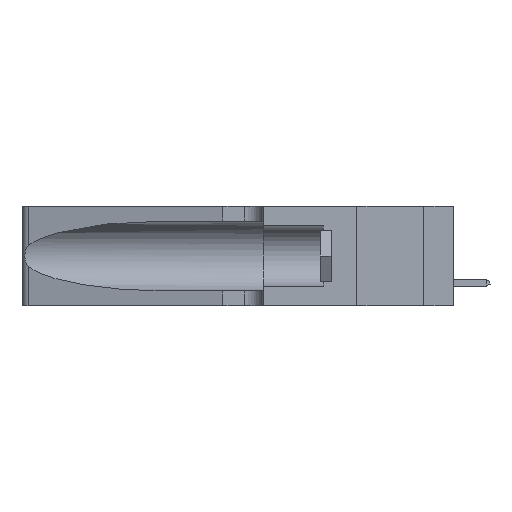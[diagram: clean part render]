
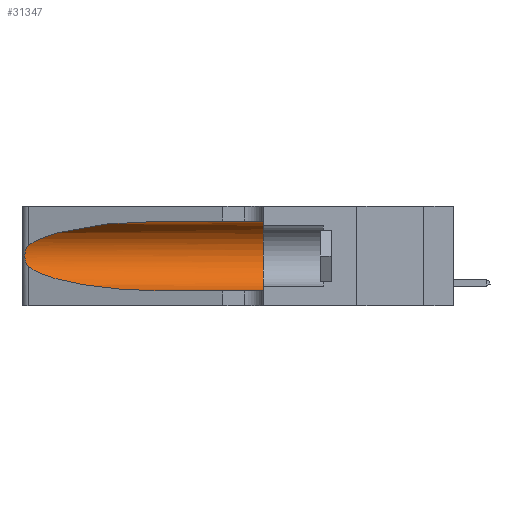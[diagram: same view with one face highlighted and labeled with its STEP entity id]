
A CAD part, left-side view. The second image highlights one B-rep face of the part: STEP entity #31347.
In plain terms, the highlighted cylindrical face has radius 3.308 mm (diameter 6.617 mm), a partial arc.
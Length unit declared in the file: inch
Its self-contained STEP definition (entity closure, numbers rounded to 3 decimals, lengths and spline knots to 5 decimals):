
#149 = CARTESIAN_POINT ( 'NONE',  ( 0.18966, 0.96281, 0.05475 ) ) ;
#315 = ORIENTED_EDGE ( 'NONE', *, *, #3881, .T. ) ;
#661 = CARTESIAN_POINT ( 'NONE',  ( 0.25487, 1.22718, 0.22369 ) ) ;
#820 = CARTESIAN_POINT ( 'NONE',  ( 0.25487, 1.22718, 0.22369 ) ) ;
#1127 = LINE ( 'NONE', #7898, #20074 ) ;
#2467 = CARTESIAN_POINT ( 'NONE',  ( 0.25487, 1.22718, 0.14631 ) ) ;
#2703 = CARTESIAN_POINT ( 'NONE',  ( 0.26075, 1.23896, 0.178 ) ) ;
#3404 = CARTESIAN_POINT ( 'NONE',  ( 0.25787, 1.23484, 0.2124 ) ) ;
#3881 = EDGE_CURVE ( 'NONE', #6513, #21899, #15709, .T. ) ;
#4022 = DIRECTION ( 'NONE',  ( 0., 0., 1. ) ) ;
#4255 = DIRECTION ( 'NONE',  ( 0., 1., 0. ) ) ;
#4300 = CARTESIAN_POINT ( 'NONE',  ( 0.26018, 1.23835, 0.19895 ) ) ;
#4351 = DIRECTION ( 'NONE',  ( 0., -1., 0. ) ) ;
#4380 = ORIENTED_EDGE ( 'NONE', *, *, #20265, .T. ) ;
#4508 = EDGE_CURVE ( 'NONE', #31505, #19445, #21516, .T. ) ;
#4590 = AXIS2_PLACEMENT_3D ( 'NONE', #14344, #4255, #4022 ) ;
#4922 = ORIENTED_EDGE ( 'NONE', *, *, #27899, .F. ) ;
#5845 = CARTESIAN_POINT ( 'NONE',  ( 0.25639, 1.23184, 0.21858 ) ) ;
#5915 = CARTESIAN_POINT ( 'NONE',  ( 0.1305, 1.61858, 0.31525 ) ) ;
#5968 = CARTESIAN_POINT ( 'NONE',  ( 0.1305, 0.72297, 0.05475 ) ) ;
#6513 = VERTEX_POINT ( 'NONE', #30532 ) ;
#6635 = VERTEX_POINT ( 'NONE', #18874 ) ;
#6839 = DIRECTION ( 'NONE',  ( 0., 0., -1. ) ) ;
#7568 = EDGE_CURVE ( 'NONE', #6635, #8553, #17215, .T. ) ;
#7696 = CARTESIAN_POINT ( 'NONE',  ( 0.25487, 1.22718, 0.14631 ) ) ;
#7898 = CARTESIAN_POINT ( 'NONE',  ( 0.1305, 1.61858, 0.05475 ) ) ;
#8404 = CARTESIAN_POINT ( 'NONE',  ( 0.25854, 1.2359, 0.20912 ) ) ;
#8553 = VERTEX_POINT ( 'NONE', #13753 ) ;
#8616 = B_SPLINE_CURVE_WITH_KNOTS ( 'NONE', 3,
 ( #820, #13294, #5845, #3404, #8404, #4300, #28411, #2703, #27311, #29543, #19996, #27419, #24541, #7696 ),
 .UNSPECIFIED., .F., .F.,
 ( 4, 2, 2, 2, 2, 2, 4 ),
 ( 0., 0.00027, 0.00053, 0.00107, 0.0016, 0.00187, 0.00214 ),
 .UNSPECIFIED. ) ;
#8793 = EDGE_CURVE ( 'NONE', #21899, #31505, #8616, .T. ) ;
#10197 = CARTESIAN_POINT ( 'NONE',  ( 0.2373, 1.15595, 0.08982 ) ) ;
#10463 = DIRECTION ( 'NONE',  ( 0., -1., 0. ) ) ;
#10739 = CARTESIAN_POINT ( 'NONE',  ( 0.2373, 1.15595, 0.28018 ) ) ;
#10974 = AXIS2_PLACEMENT_3D ( 'NONE', #14072, #4351, #6839 ) ;
#12862 = ORIENTED_EDGE ( 'NONE', *, *, #8793, .T. ) ;
#13294 = CARTESIAN_POINT ( 'NONE',  ( 0.25555, 1.22994, 0.2215 ) ) ;
#13451 = EDGE_LOOP ( 'NONE', ( #315, #12862, #25390, #4380, #28908, #4922 ) ) ;
#13461 = CARTESIAN_POINT ( 'NONE',  ( 0.18966, 0.96281, 0.31525 ) ) ;
#13753 = CARTESIAN_POINT ( 'NONE',  ( 0.1305, 0.35, 0.05475 ) ) ;
#14072 = CARTESIAN_POINT ( 'NONE',  ( 0.1305, 1.61858, 0.185 ) ) ;
#14344 = CARTESIAN_POINT ( 'NONE',  ( 0.1305, 0.35, 0.185 ) ) ;
#15302 = CARTESIAN_POINT ( 'NONE',  ( 0.1305, 0.72297, 0.05475 ) ) ;
#15709 =( BOUNDED_CURVE ( )  B_SPLINE_CURVE ( 3, ( #20693, #13461, #10739, #25969 ),
 .UNSPECIFIED., .F., .T. ) 
 B_SPLINE_CURVE_WITH_KNOTS ( ( 4, 4 ),
 ( 1.5708, 2.84003 ),
 .UNSPECIFIED. ) 
 CURVE ( )  GEOMETRIC_REPRESENTATION_ITEM ( )  RATIONAL_B_SPLINE_CURVE ( ( 1., 0.87, 0.87, 1. ) ) 
 REPRESENTATION_ITEM ( '' )  );
#17038 = CYLINDRICAL_SURFACE ( 'NONE', #10974, 0.13025 ) ;
#17215 = CIRCLE ( 'NONE', #4590, 0.13025 ) ;
#18874 = CARTESIAN_POINT ( 'NONE',  ( 0.1305, 0.35, 0.31525 ) ) ;
#19445 = VERTEX_POINT ( 'NONE', #5968 ) ;
#19622 = VECTOR ( 'NONE', #20697, 39.37008 ) ;
#19996 = CARTESIAN_POINT ( 'NONE',  ( 0.25789, 1.23486, 0.15765 ) ) ;
#20074 = VECTOR ( 'NONE', #10463, 39.37008 ) ;
#20265 = EDGE_CURVE ( 'NONE', #19445, #8553, #1127, .T. ) ;
#20354 = LINE ( 'NONE', #5915, #19622 ) ;
#20693 = CARTESIAN_POINT ( 'NONE',  ( 0.1305, 0.72297, 0.31525 ) ) ;
#20697 = DIRECTION ( 'NONE',  ( 0., -1., 0. ) ) ;
#21516 =( BOUNDED_CURVE ( )  B_SPLINE_CURVE ( 3, ( #30211, #10197, #149, #15302 ),
 .UNSPECIFIED., .F., .F. ) 
 B_SPLINE_CURVE_WITH_KNOTS ( ( 4, 4 ),
 ( 3.44316, 4.71239 ),
 .UNSPECIFIED. ) 
 CURVE ( )  GEOMETRIC_REPRESENTATION_ITEM ( )  RATIONAL_B_SPLINE_CURVE ( ( 1., 0.87, 0.87, 1. ) ) 
 REPRESENTATION_ITEM ( '' )  );
#21899 = VERTEX_POINT ( 'NONE', #661 ) ;
#22059 = FACE_OUTER_BOUND ( 'NONE', #13451, .T. ) ;
#24541 = CARTESIAN_POINT ( 'NONE',  ( 0.25555, 1.22993, 0.14849 ) ) ;
#25390 = ORIENTED_EDGE ( 'NONE', *, *, #4508, .T. ) ;
#25969 = CARTESIAN_POINT ( 'NONE',  ( 0.25487, 1.22718, 0.22369 ) ) ;
#27311 = CARTESIAN_POINT ( 'NONE',  ( 0.26017, 1.23833, 0.17102 ) ) ;
#27419 = CARTESIAN_POINT ( 'NONE',  ( 0.25639, 1.23186, 0.15144 ) ) ;
#27899 = EDGE_CURVE ( 'NONE', #6513, #6635, #20354, .T. ) ;
#28411 = CARTESIAN_POINT ( 'NONE',  ( 0.26075, 1.23896, 0.19203 ) ) ;
#28908 = ORIENTED_EDGE ( 'NONE', *, *, #7568, .F. ) ;
#29543 = CARTESIAN_POINT ( 'NONE',  ( 0.25856, 1.23593, 0.16098 ) ) ;
#30211 = CARTESIAN_POINT ( 'NONE',  ( 0.25487, 1.22718, 0.14631 ) ) ;
#30532 = CARTESIAN_POINT ( 'NONE',  ( 0.1305, 0.72297, 0.31525 ) ) ;
#31347 = ADVANCED_FACE ( 'NONE', ( #22059 ), #17038, .F. ) ;
#31505 = VERTEX_POINT ( 'NONE', #2467 ) ;
